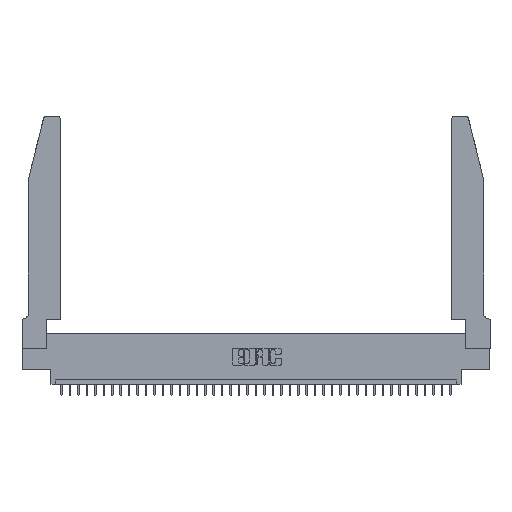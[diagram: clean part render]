
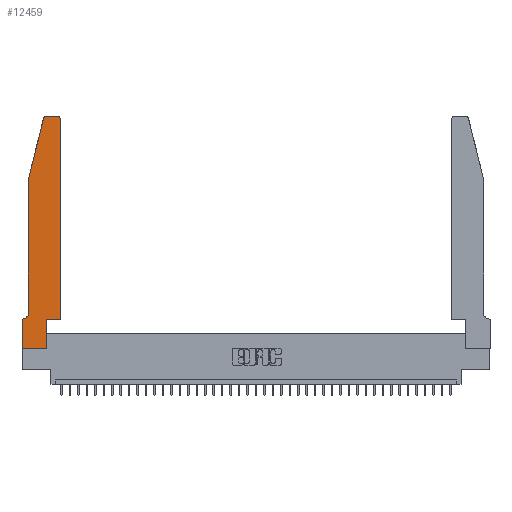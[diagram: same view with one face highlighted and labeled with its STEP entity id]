
A CAD part, top view. The second image highlights one B-rep face of the part: STEP entity #12459.
In plain terms, the highlighted planar face has unit normal (0, 0, 1).
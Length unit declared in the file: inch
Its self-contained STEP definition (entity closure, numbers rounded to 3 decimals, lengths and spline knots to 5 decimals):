
#134 = DIRECTION ( 'NONE',  ( 0., -1., 0. ) ) ;
#167 = AXIS2_PLACEMENT_3D ( 'NONE', #26661, #17420, #33473 ) ;
#1136 = CARTESIAN_POINT ( 'NONE',  ( 0.0755, 2., 0.37 ) ) ;
#1304 = VERTEX_POINT ( 'NONE', #36314 ) ;
#1673 = VERTEX_POINT ( 'NONE', #14336 ) ;
#1865 = DIRECTION ( 'NONE',  ( -1., 0., 0. ) ) ;
#1901 = VERTEX_POINT ( 'NONE', #11076 ) ;
#2925 = LINE ( 'NONE', #30055, #11346 ) ;
#2967 = VERTEX_POINT ( 'NONE', #9344 ) ;
#3272 = DIRECTION ( 'NONE',  ( 0., 0., 1. ) ) ;
#3288 = PLANE ( 'NONE',  #9650 ) ;
#3418 = LINE ( 'NONE', #37332, #30206 ) ;
#3525 = CARTESIAN_POINT ( 'NONE',  ( 0.0755, 2., 0.37 ) ) ;
#3664 = DIRECTION ( 'NONE',  ( 0., 0., 1. ) ) ;
#4049 = CARTESIAN_POINT ( 'NONE',  ( 0.284, 2.72, 0.37 ) ) ;
#4437 = CARTESIAN_POINT ( 'NONE',  ( 0.2865, 0.35, 0.37 ) ) ;
#5197 = CARTESIAN_POINT ( 'NONE',  ( 0.4505, 0.35, 0.37 ) ) ;
#5303 = EDGE_CURVE ( 'NONE', #1901, #37308, #6820, .T. ) ;
#5431 = ORIENTED_EDGE ( 'NONE', *, *, #23883, .T. ) ;
#5510 = EDGE_CURVE ( 'NONE', #14065, #34185, #32976, .T. ) ;
#5939 = EDGE_CURVE ( 'NONE', #9462, #1901, #6733, .T. ) ;
#6179 = ORIENTED_EDGE ( 'NONE', *, *, #24365, .T. ) ;
#6733 = LINE ( 'NONE', #3525, #34428 ) ;
#6820 = CIRCLE ( 'NONE', #17743, 0.07 ) ;
#9344 = CARTESIAN_POINT ( 'NONE',  ( 0., 0., 0.37 ) ) ;
#9462 = VERTEX_POINT ( 'NONE', #1136 ) ;
#9650 = AXIS2_PLACEMENT_3D ( 'NONE', #31197, #3664, #15925 ) ;
#9974 = VERTEX_POINT ( 'NONE', #17762 ) ;
#10968 = VECTOR ( 'NONE', #134, 39.37008 ) ;
#11076 = CARTESIAN_POINT ( 'NONE',  ( 0.0755, 0.42, 0.37 ) ) ;
#11346 = VECTOR ( 'NONE', #17790, 39.37008 ) ;
#11876 = CARTESIAN_POINT ( 'NONE',  ( 0.2865, 0.35, 0.37 ) ) ;
#12459 = ADVANCED_FACE ( 'NONE', ( #12894 ), #3288, .T. ) ;
#12586 = VECTOR ( 'NONE', #27168, 39.37008 ) ;
#12689 = DIRECTION ( 'NONE',  ( 1., 0., 0. ) ) ;
#12763 = LINE ( 'NONE', #31262, #25100 ) ;
#12894 = FACE_OUTER_BOUND ( 'NONE', #35175, .T. ) ;
#14017 = ORIENTED_EDGE ( 'NONE', *, *, #23773, .T. ) ;
#14065 = VERTEX_POINT ( 'NONE', #24544 ) ;
#14336 = CARTESIAN_POINT ( 'NONE',  ( 0., 0.35, 0.37 ) ) ;
#14457 = ORIENTED_EDGE ( 'NONE', *, *, #14991, .T. ) ;
#14789 = AXIS2_PLACEMENT_3D ( 'NONE', #4049, #3272, #12689 ) ;
#14991 = EDGE_CURVE ( 'NONE', #9974, #27993, #12763, .T. ) ;
#15925 = DIRECTION ( 'NONE',  ( 1., 0., 0. ) ) ;
#15975 = LINE ( 'NONE', #24438, #10968 ) ;
#17420 = DIRECTION ( 'NONE',  ( 0., 0., 1. ) ) ;
#17743 = AXIS2_PLACEMENT_3D ( 'NONE', #35193, #20537, #1865 ) ;
#17756 = CARTESIAN_POINT ( 'NONE',  ( 0.2605, 2.75, 0.37 ) ) ;
#17762 = CARTESIAN_POINT ( 'NONE',  ( 0.4505, 0.35, 0.37 ) ) ;
#17790 = DIRECTION ( 'NONE',  ( 1., 0., 0. ) ) ;
#18044 = LINE ( 'NONE', #5197, #36516 ) ;
#18568 = EDGE_CURVE ( 'NONE', #2967, #14065, #2925, .T. ) ;
#18766 = CARTESIAN_POINT ( 'NONE',  ( 0.0755, 2., 0.37 ) ) ;
#18991 = DIRECTION ( 'NONE',  ( 0., -1., 0. ) ) ;
#20537 = DIRECTION ( 'NONE',  ( 0., 0., -1. ) ) ;
#21982 = DIRECTION ( 'NONE',  ( -0.239, -0.971, 0. ) ) ;
#22623 = ORIENTED_EDGE ( 'NONE', *, *, #26337, .T. ) ;
#23770 = CARTESIAN_POINT ( 'NONE',  ( 0.284, 2.75, 0.37 ) ) ;
#23773 = EDGE_CURVE ( 'NONE', #33550, #32692, #33616, .T. ) ;
#23883 = EDGE_CURVE ( 'NONE', #32692, #1304, #30842, .T. ) ;
#24365 = EDGE_CURVE ( 'NONE', #37308, #1673, #3418, .T. ) ;
#24438 = CARTESIAN_POINT ( 'NONE',  ( 0., 0., 0.37 ) ) ;
#24544 = CARTESIAN_POINT ( 'NONE',  ( 0.2865, 0., 0.37 ) ) ;
#24712 = DIRECTION ( 'NONE',  ( -1., 0., 0. ) ) ;
#24981 = CARTESIAN_POINT ( 'NONE',  ( 0.4205, 2.75, 0.37 ) ) ;
#25100 = VECTOR ( 'NONE', #37857, 39.37008 ) ;
#26337 = EDGE_CURVE ( 'NONE', #1673, #2967, #15975, .T. ) ;
#26499 = DIRECTION ( 'NONE',  ( 1., 0., 0. ) ) ;
#26661 = CARTESIAN_POINT ( 'NONE',  ( 0.4205, 2.72, 0.37 ) ) ;
#27168 = DIRECTION ( 'NONE',  ( 0., 1., 0. ) ) ;
#27567 = EDGE_CURVE ( 'NONE', #27993, #33550, #28371, .T. ) ;
#27993 = VERTEX_POINT ( 'NONE', #34337 ) ;
#28371 = CIRCLE ( 'NONE', #167, 0.03 ) ;
#29468 = ORIENTED_EDGE ( 'NONE', *, *, #32361, .T. ) ;
#30055 = CARTESIAN_POINT ( 'NONE',  ( 0., 0., 0.37 ) ) ;
#30089 = ORIENTED_EDGE ( 'NONE', *, *, #27567, .T. ) ;
#30206 = VECTOR ( 'NONE', #24712, 39.37008 ) ;
#30842 = CIRCLE ( 'NONE', #14789, 0.03 ) ;
#31037 = ORIENTED_EDGE ( 'NONE', *, *, #5303, .T. ) ;
#31197 = CARTESIAN_POINT ( 'NONE',  ( 0., 0.35, 0.37 ) ) ;
#31262 = CARTESIAN_POINT ( 'NONE',  ( 0.4505, 0.35, 0.37 ) ) ;
#32361 = EDGE_CURVE ( 'NONE', #1304, #9462, #33836, .T. ) ;
#32692 = VERTEX_POINT ( 'NONE', #23770 ) ;
#32748 = VECTOR ( 'NONE', #36029, 39.37008 ) ;
#32976 = LINE ( 'NONE', #11876, #12586 ) ;
#33214 = ORIENTED_EDGE ( 'NONE', *, *, #5510, .T. ) ;
#33473 = DIRECTION ( 'NONE',  ( 1., 0., 0. ) ) ;
#33550 = VERTEX_POINT ( 'NONE', #24981 ) ;
#33616 = LINE ( 'NONE', #17756, #32748 ) ;
#33810 = ORIENTED_EDGE ( 'NONE', *, *, #39441, .T. ) ;
#33836 = LINE ( 'NONE', #18766, #38112 ) ;
#34185 = VERTEX_POINT ( 'NONE', #4437 ) ;
#34337 = CARTESIAN_POINT ( 'NONE',  ( 0.4505, 2.72, 0.37 ) ) ;
#34428 = VECTOR ( 'NONE', #18991, 39.37008 ) ;
#35175 = EDGE_LOOP ( 'NONE', ( #14017, #5431, #29468, #36698, #31037, #6179, #22623, #38031, #33214, #33810, #14457, #30089 ) ) ;
#35193 = CARTESIAN_POINT ( 'NONE',  ( 0.0055, 0.42, 0.37 ) ) ;
#36029 = DIRECTION ( 'NONE',  ( -1., 0., 0. ) ) ;
#36314 = CARTESIAN_POINT ( 'NONE',  ( 0.25487, 2.72718, 0.37 ) ) ;
#36516 = VECTOR ( 'NONE', #26499, 39.37008 ) ;
#36698 = ORIENTED_EDGE ( 'NONE', *, *, #5939, .T. ) ;
#37308 = VERTEX_POINT ( 'NONE', #37617 ) ;
#37332 = CARTESIAN_POINT ( 'NONE',  ( 0.0755, 0.35, 0.37 ) ) ;
#37617 = CARTESIAN_POINT ( 'NONE',  ( 0.0055, 0.35, 0.37 ) ) ;
#37857 = DIRECTION ( 'NONE',  ( 0., 1., 0. ) ) ;
#38031 = ORIENTED_EDGE ( 'NONE', *, *, #18568, .T. ) ;
#38112 = VECTOR ( 'NONE', #21982, 39.37008 ) ;
#39441 = EDGE_CURVE ( 'NONE', #34185, #9974, #18044, .T. ) ;
